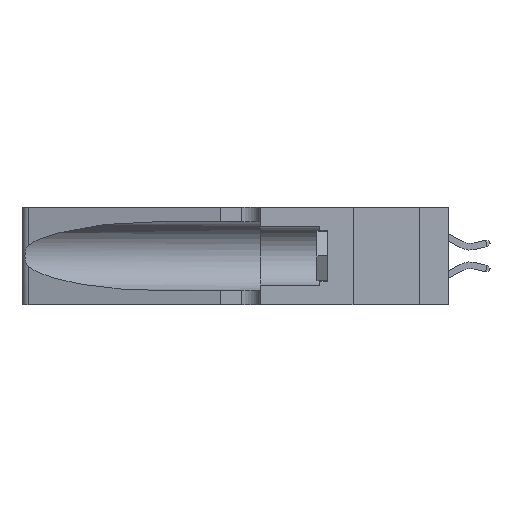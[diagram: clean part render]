
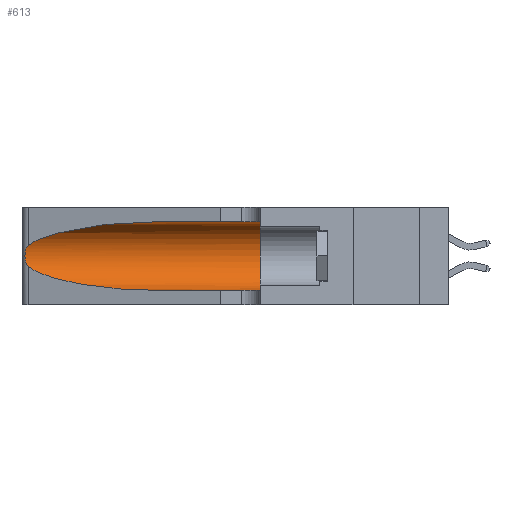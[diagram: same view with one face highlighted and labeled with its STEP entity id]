
A CAD part, left-side view. The second image highlights one B-rep face of the part: STEP entity #613.
In plain terms, the highlighted cylindrical face has radius 3.308 mm (diameter 6.617 mm), a partial arc.
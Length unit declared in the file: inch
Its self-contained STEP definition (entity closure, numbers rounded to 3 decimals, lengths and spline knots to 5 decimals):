
#214 = CARTESIAN_POINT ( 'NONE',  ( 0.25487, 1.22718, 0.22369 ) ) ;
#316 = CARTESIAN_POINT ( 'NONE',  ( 0.26075, 1.23896, 0.178 ) ) ;
#462 = CARTESIAN_POINT ( 'NONE',  ( 0.25854, 1.2359, 0.20912 ) ) ;
#613 = ADVANCED_FACE ( 'NONE', ( #17638 ), #25090, .F. ) ;
#815 = VERTEX_POINT ( 'NONE', #34842 ) ;
#1168 = EDGE_CURVE ( 'NONE', #24384, #11061, #5300, .T. ) ;
#1423 =( BOUNDED_CURVE ( )  B_SPLINE_CURVE ( 3, ( #30483, #1885, #39350, #23738 ),
 .UNSPECIFIED., .F., .T. ) 
 B_SPLINE_CURVE_WITH_KNOTS ( ( 4, 4 ),
 ( 3.44316, 4.71239 ),
 .UNSPECIFIED. ) 
 CURVE ( )  GEOMETRIC_REPRESENTATION_ITEM ( )  RATIONAL_B_SPLINE_CURVE ( ( 1., 0.87, 0.87, 1. ) ) 
 REPRESENTATION_ITEM ( '' )  );
#1560 = CARTESIAN_POINT ( 'NONE',  ( 0.1305, 0.72297, 0.05475 ) ) ;
#1885 = CARTESIAN_POINT ( 'NONE',  ( 0.2373, 1.15595, 0.08982 ) ) ;
#1939 = CARTESIAN_POINT ( 'NONE',  ( 0.25487, 1.22718, 0.14631 ) ) ;
#1981 = DIRECTION ( 'NONE',  ( 0., -1., 0. ) ) ;
#2764 = DIRECTION ( 'NONE',  ( 0., 1., 0. ) ) ;
#4093 = CARTESIAN_POINT ( 'NONE',  ( 0.26017, 1.23833, 0.17102 ) ) ;
#4969 = CARTESIAN_POINT ( 'NONE',  ( 0.1305, 1.61858, 0.31525 ) ) ;
#5258 = CARTESIAN_POINT ( 'NONE',  ( 0.1305, 1.61858, 0.05475 ) ) ;
#5300 = LINE ( 'NONE', #5258, #19071 ) ;
#5366 = CARTESIAN_POINT ( 'NONE',  ( 0.25789, 1.23486, 0.15765 ) ) ;
#5377 = CARTESIAN_POINT ( 'NONE',  ( 0.25639, 1.23186, 0.15144 ) ) ;
#6397 = CARTESIAN_POINT ( 'NONE',  ( 0.26018, 1.23835, 0.19895 ) ) ;
#7480 = CARTESIAN_POINT ( 'NONE',  ( 0.1305, 0.35, 0.05475 ) ) ;
#7703 = CARTESIAN_POINT ( 'NONE',  ( 0.1305, 1.61858, 0.185 ) ) ;
#7783 = CARTESIAN_POINT ( 'NONE',  ( 0.18966, 0.96281, 0.31525 ) ) ;
#10976 = VERTEX_POINT ( 'NONE', #27096 ) ;
#10990 = EDGE_CURVE ( 'NONE', #25425, #11061, #12861, .T. ) ;
#11061 = VERTEX_POINT ( 'NONE', #7480 ) ;
#12087 = EDGE_CURVE ( 'NONE', #25396, #24384, #1423, .T. ) ;
#12220 = LINE ( 'NONE', #4969, #37793 ) ;
#12335 = CARTESIAN_POINT ( 'NONE',  ( 0.26075, 1.23896, 0.19203 ) ) ;
#12630 = ORIENTED_EDGE ( 'NONE', *, *, #30204, .T. ) ;
#12861 = CIRCLE ( 'NONE', #32594, 0.13025 ) ;
#13042 = ORIENTED_EDGE ( 'NONE', *, *, #12087, .T. ) ;
#14356 = DIRECTION ( 'NONE',  ( 0., 0., -1. ) ) ;
#14725 = CARTESIAN_POINT ( 'NONE',  ( 0.25487, 1.22718, 0.14631 ) ) ;
#15497 = B_SPLINE_CURVE_WITH_KNOTS ( 'NONE', 3,
 ( #214, #32040, #28345, #25303, #462, #6397, #12335, #316, #4093, #28099, #5366, #5377, #27256, #1939 ),
 .UNSPECIFIED., .F., .F.,
 ( 4, 2, 2, 2, 2, 2, 4 ),
 ( 0., 0.00027, 0.00053, 0.00107, 0.0016, 0.00187, 0.00214 ),
 .UNSPECIFIED. ) ;
#17638 = FACE_OUTER_BOUND ( 'NONE', #33029, .T. ) ;
#19071 = VECTOR ( 'NONE', #37118, 39.37008 ) ;
#22162 = ORIENTED_EDGE ( 'NONE', *, *, #27879, .T. ) ;
#23738 = CARTESIAN_POINT ( 'NONE',  ( 0.1305, 0.72297, 0.05475 ) ) ;
#24384 = VERTEX_POINT ( 'NONE', #1560 ) ;
#25090 = CYLINDRICAL_SURFACE ( 'NONE', #27315, 0.13025 ) ;
#25303 = CARTESIAN_POINT ( 'NONE',  ( 0.25787, 1.23484, 0.2124 ) ) ;
#25396 = VERTEX_POINT ( 'NONE', #14725 ) ;
#25425 = VERTEX_POINT ( 'NONE', #32985 ) ;
#26263 = CARTESIAN_POINT ( 'NONE',  ( 0.2373, 1.15595, 0.28018 ) ) ;
#26412 = CARTESIAN_POINT ( 'NONE',  ( 0.1305, 0.72297, 0.31525 ) ) ;
#27096 = CARTESIAN_POINT ( 'NONE',  ( 0.25487, 1.22718, 0.22369 ) ) ;
#27256 = CARTESIAN_POINT ( 'NONE',  ( 0.25555, 1.22993, 0.14849 ) ) ;
#27315 = AXIS2_PLACEMENT_3D ( 'NONE', #7703, #36869, #14356 ) ;
#27879 = EDGE_CURVE ( 'NONE', #815, #10976, #33888, .T. ) ;
#28099 = CARTESIAN_POINT ( 'NONE',  ( 0.25856, 1.23593, 0.16098 ) ) ;
#28345 = CARTESIAN_POINT ( 'NONE',  ( 0.25639, 1.23184, 0.21858 ) ) ;
#28781 = DIRECTION ( 'NONE',  ( 0., 0., 1. ) ) ;
#29445 = CARTESIAN_POINT ( 'NONE',  ( 0.25487, 1.22718, 0.22369 ) ) ;
#30204 = EDGE_CURVE ( 'NONE', #10976, #25396, #15497, .T. ) ;
#30483 = CARTESIAN_POINT ( 'NONE',  ( 0.25487, 1.22718, 0.14631 ) ) ;
#32040 = CARTESIAN_POINT ( 'NONE',  ( 0.25555, 1.22994, 0.2215 ) ) ;
#32594 = AXIS2_PLACEMENT_3D ( 'NONE', #34302, #2764, #28781 ) ;
#32655 = ORIENTED_EDGE ( 'NONE', *, *, #1168, .T. ) ;
#32985 = CARTESIAN_POINT ( 'NONE',  ( 0.1305, 0.35, 0.31525 ) ) ;
#33029 = EDGE_LOOP ( 'NONE', ( #22162, #12630, #13042, #32655, #34942, #38901 ) ) ;
#33888 =( BOUNDED_CURVE ( )  B_SPLINE_CURVE ( 3, ( #26412, #7783, #26263, #29445 ),
 .UNSPECIFIED., .F., .T. ) 
 B_SPLINE_CURVE_WITH_KNOTS ( ( 4, 4 ),
 ( 1.5708, 2.84003 ),
 .UNSPECIFIED. ) 
 CURVE ( )  GEOMETRIC_REPRESENTATION_ITEM ( )  RATIONAL_B_SPLINE_CURVE ( ( 1., 0.87, 0.87, 1. ) ) 
 REPRESENTATION_ITEM ( '' )  );
#34302 = CARTESIAN_POINT ( 'NONE',  ( 0.1305, 0.35, 0.185 ) ) ;
#34719 = EDGE_CURVE ( 'NONE', #815, #25425, #12220, .T. ) ;
#34842 = CARTESIAN_POINT ( 'NONE',  ( 0.1305, 0.72297, 0.31525 ) ) ;
#34942 = ORIENTED_EDGE ( 'NONE', *, *, #10990, .F. ) ;
#36869 = DIRECTION ( 'NONE',  ( 0., -1., 0. ) ) ;
#37118 = DIRECTION ( 'NONE',  ( 0., -1., 0. ) ) ;
#37793 = VECTOR ( 'NONE', #1981, 39.37008 ) ;
#38901 = ORIENTED_EDGE ( 'NONE', *, *, #34719, .F. ) ;
#39350 = CARTESIAN_POINT ( 'NONE',  ( 0.18966, 0.96281, 0.05475 ) ) ;
